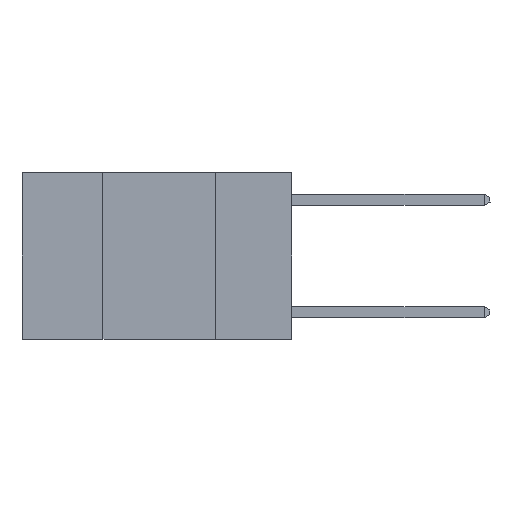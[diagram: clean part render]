
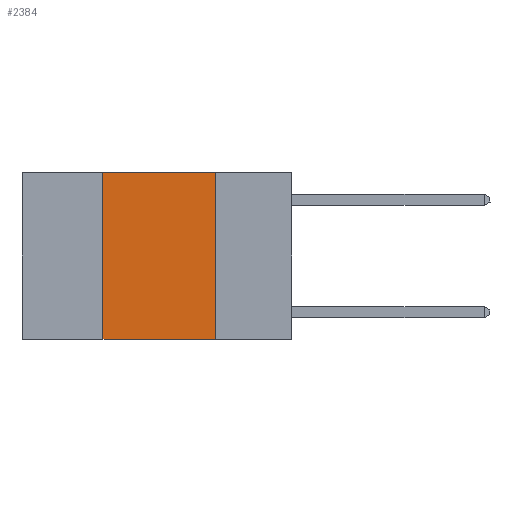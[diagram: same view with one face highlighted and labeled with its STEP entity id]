
A CAD part, left-side view. The second image highlights one B-rep face of the part: STEP entity #2384.
In plain terms, the highlighted planar face has unit normal (-1, 0, 0).
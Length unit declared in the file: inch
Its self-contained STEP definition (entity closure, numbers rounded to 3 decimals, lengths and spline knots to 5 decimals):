
#77 = DIRECTION ( 'NONE',  ( 0., -1., 0. ) ) ;
#408 = CARTESIAN_POINT ( 'NONE',  ( 0., 0.17, 0. ) ) ;
#1082 = EDGE_CURVE ( 'NONE', #13446, #1758, #11178, .T. ) ;
#1506 = EDGE_LOOP ( 'NONE', ( #9628, #10711, #2533, #9243 ) ) ;
#1758 = VERTEX_POINT ( 'NONE', #7336 ) ;
#2323 = VERTEX_POINT ( 'NONE', #7587 ) ;
#2384 = ADVANCED_FACE ( 'NONE', ( #6010 ), #12067, .F. ) ;
#2500 = CARTESIAN_POINT ( 'NONE',  ( 0., 0.42, -0.37 ) ) ;
#2533 = ORIENTED_EDGE ( 'NONE', *, *, #1082, .F. ) ;
#3078 = DIRECTION ( 'NONE',  ( 0., -1., 0. ) ) ;
#3483 = EDGE_CURVE ( 'NONE', #1758, #2323, #9726, .T. ) ;
#4170 = DIRECTION ( 'NONE',  ( 0., 0., 1. ) ) ;
#4687 = LINE ( 'NONE', #408, #10548 ) ;
#5942 = CARTESIAN_POINT ( 'NONE',  ( 0., 0.42, 0. ) ) ;
#6010 = FACE_OUTER_BOUND ( 'NONE', #1506, .T. ) ;
#6272 = AXIS2_PLACEMENT_3D ( 'NONE', #13510, #11989, #11893 ) ;
#6653 = VERTEX_POINT ( 'NONE', #12624 ) ;
#7336 = CARTESIAN_POINT ( 'NONE',  ( 0., 0.42, 0. ) ) ;
#7587 = CARTESIAN_POINT ( 'NONE',  ( 0., 0.17, 0. ) ) ;
#9153 = EDGE_CURVE ( 'NONE', #2323, #6653, #4687, .T. ) ;
#9243 = ORIENTED_EDGE ( 'NONE', *, *, #9619, .T. ) ;
#9619 = EDGE_CURVE ( 'NONE', #13446, #6653, #14003, .T. ) ;
#9628 = ORIENTED_EDGE ( 'NONE', *, *, #9153, .F. ) ;
#9726 = LINE ( 'NONE', #12645, #11929 ) ;
#9740 = CARTESIAN_POINT ( 'NONE',  ( 0., 0.6, -0.37 ) ) ;
#10509 = VECTOR ( 'NONE', #4170, 39.37008 ) ;
#10548 = VECTOR ( 'NONE', #10799, 39.37008 ) ;
#10711 = ORIENTED_EDGE ( 'NONE', *, *, #3483, .F. ) ;
#10799 = DIRECTION ( 'NONE',  ( 0., 0., -1. ) ) ;
#11178 = LINE ( 'NONE', #5942, #10509 ) ;
#11893 = DIRECTION ( 'NONE',  ( 0., 0., -1. ) ) ;
#11929 = VECTOR ( 'NONE', #77, 39.37008 ) ;
#11989 = DIRECTION ( 'NONE',  ( 1., 0., 0. ) ) ;
#12067 = PLANE ( 'NONE',  #6272 ) ;
#12624 = CARTESIAN_POINT ( 'NONE',  ( 0., 0.17, -0.37 ) ) ;
#12645 = CARTESIAN_POINT ( 'NONE',  ( 0., 0.6, 0. ) ) ;
#13446 = VERTEX_POINT ( 'NONE', #2500 ) ;
#13510 = CARTESIAN_POINT ( 'NONE',  ( 0., 0.6, 0. ) ) ;
#13693 = VECTOR ( 'NONE', #3078, 39.37008 ) ;
#14003 = LINE ( 'NONE', #9740, #13693 ) ;
